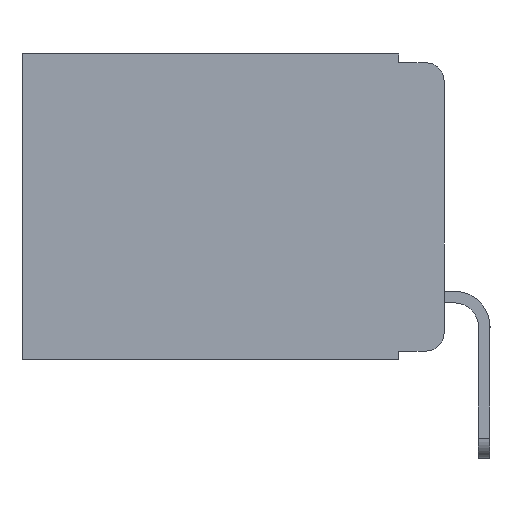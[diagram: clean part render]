
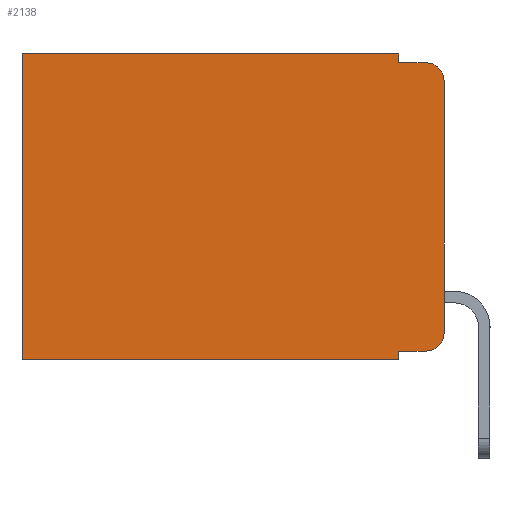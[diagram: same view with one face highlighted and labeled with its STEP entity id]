
A CAD part, left-side view. The second image highlights one B-rep face of the part: STEP entity #2138.
In plain terms, the highlighted planar face has unit normal (-1, 0, 0).
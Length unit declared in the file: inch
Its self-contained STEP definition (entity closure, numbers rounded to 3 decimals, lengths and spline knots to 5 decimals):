
#169 = CARTESIAN_POINT ( 'NONE',  ( 0.298, 0.051, 0. ) ) ;
#333 = EDGE_CURVE ( 'NONE', #2395, #8816, #9263, .T. ) ;
#385 = CARTESIAN_POINT ( 'NONE',  ( 0.298, 0., 0. ) ) ;
#478 = CIRCLE ( 'NONE', #731, 0.02 ) ;
#535 = VERTEX_POINT ( 'NONE', #13408 ) ;
#573 = EDGE_CURVE ( 'NONE', #1107, #9883, #11037, .T. ) ;
#731 = AXIS2_PLACEMENT_3D ( 'NONE', #11790, #3343, #757 ) ;
#750 = DIRECTION ( 'NONE',  ( 0., 1., 0. ) ) ;
#753 = VERTEX_POINT ( 'NONE', #1038 ) ;
#757 = DIRECTION ( 'NONE',  ( 0., 0., -1. ) ) ;
#788 = ORIENTED_EDGE ( 'NONE', *, *, #10538, .T. ) ;
#806 = ORIENTED_EDGE ( 'NONE', *, *, #11562, .T. ) ;
#1038 = CARTESIAN_POINT ( 'NONE',  ( 0.298, 0.02, -0.01 ) ) ;
#1107 = VERTEX_POINT ( 'NONE', #1845 ) ;
#1154 = VECTOR ( 'NONE', #750, 39.37008 ) ;
#1403 = DIRECTION ( 'NONE',  ( 0., 0., -1. ) ) ;
#1626 = CARTESIAN_POINT ( 'NONE',  ( 0.298, 0.051, -0.343 ) ) ;
#1845 = CARTESIAN_POINT ( 'NONE',  ( 0.298, 0.051, 0. ) ) ;
#2138 = ADVANCED_FACE ( 'NONE', ( #15989 ), #11104, .F. ) ;
#2353 = CARTESIAN_POINT ( 'NONE',  ( 0.298, 0., 0. ) ) ;
#2395 = VERTEX_POINT ( 'NONE', #1626 ) ;
#2475 = ORIENTED_EDGE ( 'NONE', *, *, #14225, .T. ) ;
#2513 = DIRECTION ( 'NONE',  ( 0., 0., -1. ) ) ;
#2528 = ORIENTED_EDGE ( 'NONE', *, *, #333, .F. ) ;
#2841 = LINE ( 'NONE', #12511, #6626 ) ;
#2872 = EDGE_CURVE ( 'NONE', #3051, #753, #478, .T. ) ;
#3051 = VERTEX_POINT ( 'NONE', #7116 ) ;
#3064 = DIRECTION ( 'NONE',  ( 0., -1., 0. ) ) ;
#3251 = DIRECTION ( 'NONE',  ( 0., 0., -1. ) ) ;
#3343 = DIRECTION ( 'NONE',  ( -1., 0., 0. ) ) ;
#3826 = DIRECTION ( 'NONE',  ( 0., -1., 0. ) ) ;
#3876 = CARTESIAN_POINT ( 'NONE',  ( 0.298, 0.051, -0.01 ) ) ;
#4296 = EDGE_CURVE ( 'NONE', #3051, #10881, #6613, .T. ) ;
#4576 = ORIENTED_EDGE ( 'NONE', *, *, #14701, .F. ) ;
#4736 = ORIENTED_EDGE ( 'NONE', *, *, #2872, .T. ) ;
#5528 = CARTESIAN_POINT ( 'NONE',  ( 0.298, 0.473, 0. ) ) ;
#6244 = LINE ( 'NONE', #169, #15150 ) ;
#6493 = CARTESIAN_POINT ( 'NONE',  ( 0.298, 0.051, 0. ) ) ;
#6613 = LINE ( 'NONE', #385, #7519 ) ;
#6626 = VECTOR ( 'NONE', #3826, 39.37008 ) ;
#6671 = LINE ( 'NONE', #10410, #8837 ) ;
#6898 = LINE ( 'NONE', #5528, #7176 ) ;
#7116 = CARTESIAN_POINT ( 'NONE',  ( 0.298, 0., -0.03 ) ) ;
#7176 = VECTOR ( 'NONE', #3251, 39.37008 ) ;
#7284 = CARTESIAN_POINT ( 'NONE',  ( 0.298, 0., -0.313 ) ) ;
#7430 = CARTESIAN_POINT ( 'NONE',  ( 0.298, 0.02, -0.333 ) ) ;
#7519 = VECTOR ( 'NONE', #7906, 39.37008 ) ;
#7906 = DIRECTION ( 'NONE',  ( 0., 0., -1. ) ) ;
#8520 = ORIENTED_EDGE ( 'NONE', *, *, #13813, .F. ) ;
#8635 = VECTOR ( 'NONE', #3064, 39.37008 ) ;
#8711 = ORIENTED_EDGE ( 'NONE', *, *, #9148, .T. ) ;
#8816 = VERTEX_POINT ( 'NONE', #14323 ) ;
#8837 = VECTOR ( 'NONE', #9201, 39.37008 ) ;
#9148 = EDGE_CURVE ( 'NONE', #14670, #10953, #2841, .T. ) ;
#9201 = DIRECTION ( 'NONE',  ( 0., 1., 0. ) ) ;
#9208 = EDGE_LOOP ( 'NONE', ( #14592, #4736, #8520, #11096, #806, #788, #2528, #4576, #8711, #2475 ) ) ;
#9263 = LINE ( 'NONE', #12916, #1154 ) ;
#9309 = DIRECTION ( 'NONE',  ( 0., 0., -1. ) ) ;
#9325 = LINE ( 'NONE', #14202, #8635 ) ;
#9883 = VERTEX_POINT ( 'NONE', #3876 ) ;
#10195 = AXIS2_PLACEMENT_3D ( 'NONE', #12883, #11978, #9309 ) ;
#10410 = CARTESIAN_POINT ( 'NONE',  ( 0.298, 0., 0. ) ) ;
#10445 = CIRCLE ( 'NONE', #10195, 0.02 ) ;
#10538 = EDGE_CURVE ( 'NONE', #535, #8816, #6898, .T. ) ;
#10881 = VERTEX_POINT ( 'NONE', #7284 ) ;
#10953 = VERTEX_POINT ( 'NONE', #7430 ) ;
#11037 = LINE ( 'NONE', #6493, #13609 ) ;
#11096 = ORIENTED_EDGE ( 'NONE', *, *, #573, .F. ) ;
#11104 = PLANE ( 'NONE',  #11615 ) ;
#11116 = CARTESIAN_POINT ( 'NONE',  ( 0.298, 0.051, -0.333 ) ) ;
#11562 = EDGE_CURVE ( 'NONE', #1107, #535, #6671, .T. ) ;
#11615 = AXIS2_PLACEMENT_3D ( 'NONE', #2353, #12248, #2513 ) ;
#11790 = CARTESIAN_POINT ( 'NONE',  ( 0.298, 0.02, -0.03 ) ) ;
#11978 = DIRECTION ( 'NONE',  ( -1., 0., 0. ) ) ;
#12248 = DIRECTION ( 'NONE',  ( 1., 0., 0. ) ) ;
#12338 = DIRECTION ( 'NONE',  ( 0., 0., -1. ) ) ;
#12511 = CARTESIAN_POINT ( 'NONE',  ( 0.298, 0.051, -0.333 ) ) ;
#12883 = CARTESIAN_POINT ( 'NONE',  ( 0.298, 0.02, -0.313 ) ) ;
#12916 = CARTESIAN_POINT ( 'NONE',  ( 0.298, 0., -0.343 ) ) ;
#13408 = CARTESIAN_POINT ( 'NONE',  ( 0.298, 0.473, 0. ) ) ;
#13609 = VECTOR ( 'NONE', #1403, 39.37008 ) ;
#13813 = EDGE_CURVE ( 'NONE', #9883, #753, #9325, .T. ) ;
#14202 = CARTESIAN_POINT ( 'NONE',  ( 0.298, 0.051, -0.01 ) ) ;
#14225 = EDGE_CURVE ( 'NONE', #10953, #10881, #10445, .T. ) ;
#14323 = CARTESIAN_POINT ( 'NONE',  ( 0.298, 0.473, -0.343 ) ) ;
#14592 = ORIENTED_EDGE ( 'NONE', *, *, #4296, .F. ) ;
#14670 = VERTEX_POINT ( 'NONE', #11116 ) ;
#14701 = EDGE_CURVE ( 'NONE', #14670, #2395, #6244, .T. ) ;
#15150 = VECTOR ( 'NONE', #12338, 39.37008 ) ;
#15989 = FACE_OUTER_BOUND ( 'NONE', #9208, .T. ) ;
